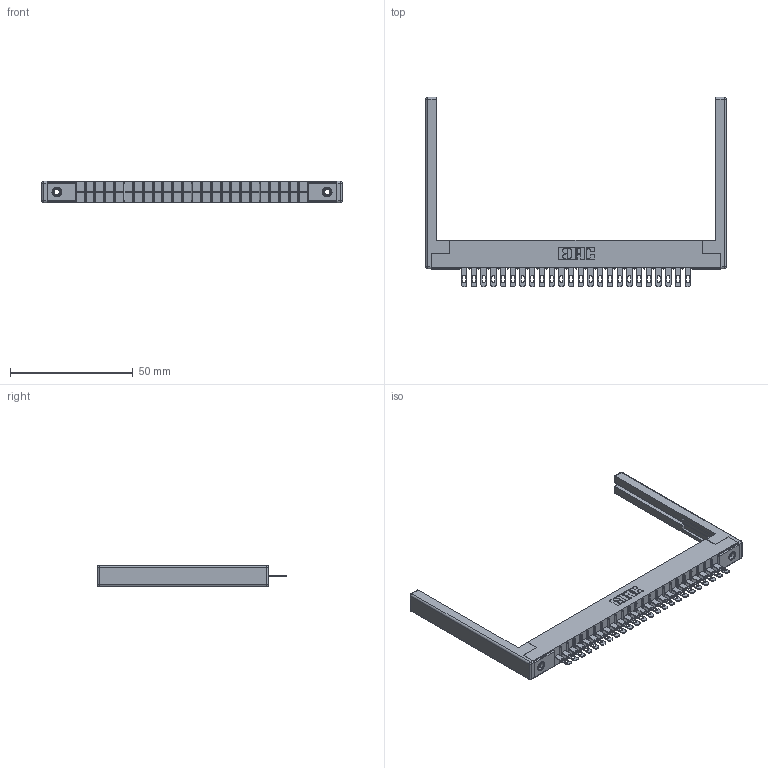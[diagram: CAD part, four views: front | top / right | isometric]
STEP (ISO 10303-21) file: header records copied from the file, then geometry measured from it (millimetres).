
FILE_DESCRIPTION (( 'STEP AP203' ), '1' );
FILE_NAME ('306-024-400-168.STEP', '2020-09-21T22:09:38', ( '' ), ( '' ), 'SwSTEP 2.0', 'SolidWorks 2020', '' );
FILE_SCHEMA (( 'CONFIG_CONTROL_DESIGN' ));
Length unit declared in the file: inch
Products named in the file (5): 306-290-001_100; 306-024-400-168; 306 Part_.156 Dia; 345-250-001_345-250-001-102; 307-220-068
Assembly tree (29 placements, depth 2):
  306-024-400-168
    306 Part_.156 Dia
    306-290-001_100  x24
    345-250-001_345-250-001-102  x2
    307-220-068  x2
Bounding box: 122.53 x 77.17 x 8.71 mm (x, y, z)
Volume: 13010.4 mm3; surface area: 17078.1 mm2
Topology: 29 solids, 29 shells, 2094 faces, 5866 edges, 3760 vertices
Faces by surface type: plane 1356, cylinder 618, sphere 104, cone 12, torus 4
Entity records: 27636 total; most frequent: CARTESIAN_POINT 4604, DIRECTION 4555, ORIENTED_EDGE 4554, EDGE_CURVE 2277, LINE 1765, VECTOR 1765, VERTEX_POINT 1444, AXIS2_PLACEMENT_3D 1395
